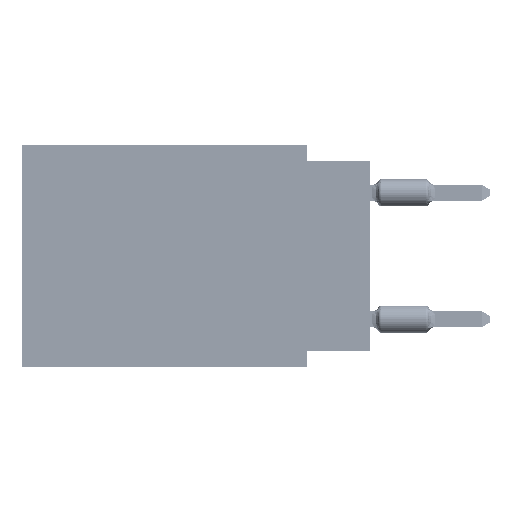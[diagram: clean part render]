
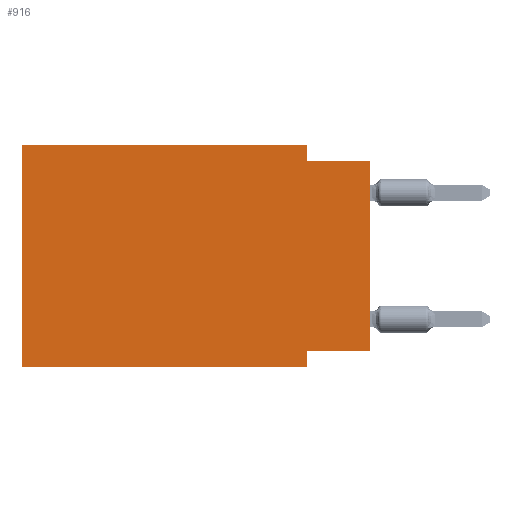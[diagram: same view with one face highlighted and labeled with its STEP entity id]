
A CAD part, left-side view. The second image highlights one B-rep face of the part: STEP entity #916.
In plain terms, the highlighted planar face has unit normal (-1, 0, 0).
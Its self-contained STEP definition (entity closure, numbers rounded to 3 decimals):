
#560 = VECTOR ( 'NONE', #51160, 1000. ) ;
#916 = ADVANCED_FACE ( 'NONE', ( #43614 ), #84267, .F. ) ;
#3669 = CARTESIAN_POINT ( 'NONE',  ( 0., 2.54, 0. ) ) ;
#4294 = VECTOR ( 'NONE', #69188, 1000. ) ;
#5169 = LINE ( 'NONE', #44905, #29700 ) ;
#8264 = VERTEX_POINT ( 'NONE', #76206 ) ;
#9361 = LINE ( 'NONE', #24226, #40340 ) ;
#10948 = ORIENTED_EDGE ( 'NONE', *, *, #68555, .F. ) ;
#12993 = CARTESIAN_POINT ( 'NONE',  ( 0., 0., -0.635 ) ) ;
#16748 = DIRECTION ( 'NONE',  ( 0., -1., 0. ) ) ;
#17654 = EDGE_CURVE ( 'NONE', #22259, #8264, #48869, .T. ) ;
#17981 = VERTEX_POINT ( 'NONE', #3669 ) ;
#18260 = DIRECTION ( 'NONE',  ( 0., -1., 0. ) ) ;
#19777 = LINE ( 'NONE', #61779, #80564 ) ;
#21076 = DIRECTION ( 'NONE',  ( 1., 0., 0. ) ) ;
#21192 = ORIENTED_EDGE ( 'NONE', *, *, #46051, .F. ) ;
#21372 = ORIENTED_EDGE ( 'NONE', *, *, #17654, .F. ) ;
#22012 = ORIENTED_EDGE ( 'NONE', *, *, #77831, .T. ) ;
#22259 = VERTEX_POINT ( 'NONE', #26736 ) ;
#23522 = CARTESIAN_POINT ( 'NONE',  ( 0., 0., -0.635 ) ) ;
#24226 = CARTESIAN_POINT ( 'NONE',  ( 0., 2.54, -8.89 ) ) ;
#26736 = CARTESIAN_POINT ( 'NONE',  ( 0., 13.97, -8.89 ) ) ;
#27196 = CARTESIAN_POINT ( 'NONE',  ( 0., 0., 0. ) ) ;
#28266 = EDGE_CURVE ( 'NONE', #8264, #17981, #49836, .T. ) ;
#29051 = EDGE_CURVE ( 'NONE', #61820, #64107, #33062, .T. ) ;
#29700 = VECTOR ( 'NONE', #18260, 1000. ) ;
#31517 = EDGE_CURVE ( 'NONE', #77037, #64107, #65054, .T. ) ;
#32001 = CARTESIAN_POINT ( 'NONE',  ( 0., 2.54, -0.635 ) ) ;
#33062 = LINE ( 'NONE', #27196, #71304 ) ;
#33540 = CARTESIAN_POINT ( 'NONE',  ( 0., 13.97, 0. ) ) ;
#34053 = EDGE_LOOP ( 'NONE', ( #70647, #62700, #10948, #67997, #21372, #22012, #21192, #80891 ) ) ;
#36413 = DIRECTION ( 'NONE',  ( 0., 0., -1. ) ) ;
#36453 = AXIS2_PLACEMENT_3D ( 'NONE', #55425, #21076, #36413 ) ;
#40340 = VECTOR ( 'NONE', #86065, 1000. ) ;
#41699 = CARTESIAN_POINT ( 'NONE',  ( 0., 2.54, -8.255 ) ) ;
#43614 = FACE_OUTER_BOUND ( 'NONE', #34053, .T. ) ;
#44905 = CARTESIAN_POINT ( 'NONE',  ( 0., 13.97, -8.89 ) ) ;
#46051 = EDGE_CURVE ( 'NONE', #48155, #53712, #9361, .T. ) ;
#46168 = DIRECTION ( 'NONE',  ( 0., 0., 1. ) ) ;
#48155 = VERTEX_POINT ( 'NONE', #41699 ) ;
#48869 = LINE ( 'NONE', #33540, #4294 ) ;
#49777 = VECTOR ( 'NONE', #16748, 1000. ) ;
#49836 = LINE ( 'NONE', #50279, #560 ) ;
#50279 = CARTESIAN_POINT ( 'NONE',  ( 0., 13.97, 0. ) ) ;
#51160 = DIRECTION ( 'NONE',  ( 0., -1., 0. ) ) ;
#51338 = LINE ( 'NONE', #86976, #65964 ) ;
#53712 = VERTEX_POINT ( 'NONE', #62064 ) ;
#55425 = CARTESIAN_POINT ( 'NONE',  ( 0., 13.97, 0. ) ) ;
#57158 = EDGE_CURVE ( 'NONE', #61820, #48155, #19777, .T. ) ;
#61779 = CARTESIAN_POINT ( 'NONE',  ( 0., 0., -8.255 ) ) ;
#61820 = VERTEX_POINT ( 'NONE', #65120 ) ;
#62064 = CARTESIAN_POINT ( 'NONE',  ( 0., 2.54, -8.89 ) ) ;
#62700 = ORIENTED_EDGE ( 'NONE', *, *, #31517, .F. ) ;
#64107 = VERTEX_POINT ( 'NONE', #12993 ) ;
#65054 = LINE ( 'NONE', #23522, #49777 ) ;
#65120 = CARTESIAN_POINT ( 'NONE',  ( 0., 0., -8.255 ) ) ;
#65964 = VECTOR ( 'NONE', #72555, 1000. ) ;
#67997 = ORIENTED_EDGE ( 'NONE', *, *, #28266, .F. ) ;
#68555 = EDGE_CURVE ( 'NONE', #17981, #77037, #51338, .T. ) ;
#69188 = DIRECTION ( 'NONE',  ( 0., 0., 1. ) ) ;
#70647 = ORIENTED_EDGE ( 'NONE', *, *, #29051, .T. ) ;
#71304 = VECTOR ( 'NONE', #46168, 1000. ) ;
#72555 = DIRECTION ( 'NONE',  ( 0., 0., -1. ) ) ;
#74870 = DIRECTION ( 'NONE',  ( 0., 1., 0. ) ) ;
#76206 = CARTESIAN_POINT ( 'NONE',  ( 0., 13.97, 0. ) ) ;
#77037 = VERTEX_POINT ( 'NONE', #32001 ) ;
#77831 = EDGE_CURVE ( 'NONE', #22259, #53712, #5169, .T. ) ;
#80564 = VECTOR ( 'NONE', #74870, 1000. ) ;
#80891 = ORIENTED_EDGE ( 'NONE', *, *, #57158, .F. ) ;
#84267 = PLANE ( 'NONE',  #36453 ) ;
#86065 = DIRECTION ( 'NONE',  ( 0., 0., -1. ) ) ;
#86976 = CARTESIAN_POINT ( 'NONE',  ( 0., 2.54, 0. ) ) ;
